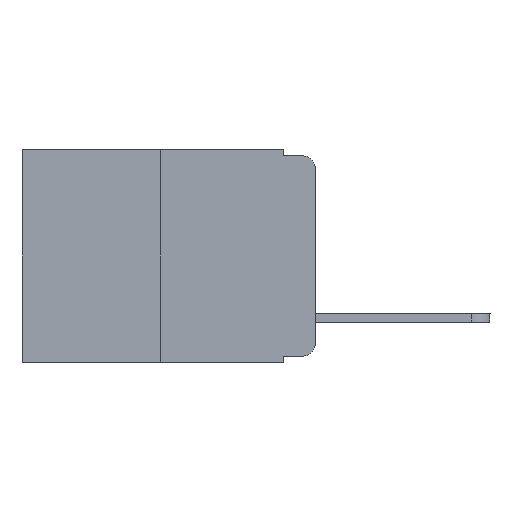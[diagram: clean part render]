
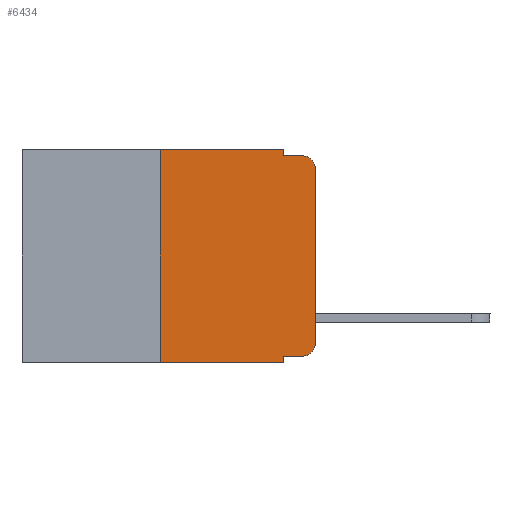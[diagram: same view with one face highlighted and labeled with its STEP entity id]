
A CAD part, left-side view. The second image highlights one B-rep face of the part: STEP entity #6434.
In plain terms, the highlighted planar face has unit normal (-1, 0, 0).
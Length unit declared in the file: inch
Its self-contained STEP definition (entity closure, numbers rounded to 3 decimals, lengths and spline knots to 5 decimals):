
#487 = DIRECTION ( 'NONE',  ( 0., -1., 0. ) ) ;
#492 = EDGE_CURVE ( 'NONE', #10321, #3591, #4329, .T. ) ;
#918 = VERTEX_POINT ( 'NONE', #18672 ) ;
#949 = EDGE_CURVE ( 'NONE', #10948, #1924, #9580, .T. ) ;
#983 = DIRECTION ( 'NONE',  ( 0., -1., 0. ) ) ;
#1165 = ORIENTED_EDGE ( 'NONE', *, *, #949, .T. ) ;
#1637 = CARTESIAN_POINT ( 'NONE',  ( 0., 0.473, -0.343 ) ) ;
#1924 = VERTEX_POINT ( 'NONE', #9732 ) ;
#2140 = AXIS2_PLACEMENT_3D ( 'NONE', #17310, #14210, #14512 ) ;
#2170 = DIRECTION ( 'NONE',  ( 0., -1., 0. ) ) ;
#2249 = DIRECTION ( 'NONE',  ( 1., 0., 0. ) ) ;
#2569 = LINE ( 'NONE', #8478, #4592 ) ;
#2744 = VECTOR ( 'NONE', #487, 39.37008 ) ;
#2855 = CARTESIAN_POINT ( 'NONE',  ( 0., 0.051, 0. ) ) ;
#3085 = ORIENTED_EDGE ( 'NONE', *, *, #8043, .F. ) ;
#3117 = ORIENTED_EDGE ( 'NONE', *, *, #14509, .F. ) ;
#3208 = LINE ( 'NONE', #7824, #2744 ) ;
#3591 = VERTEX_POINT ( 'NONE', #11490 ) ;
#3727 = LINE ( 'NONE', #6775, #8864 ) ;
#3771 = DIRECTION ( 'NONE',  ( 0., -1., 0. ) ) ;
#3957 = LINE ( 'NONE', #9946, #10611 ) ;
#4056 = EDGE_CURVE ( 'NONE', #10321, #16204, #3208, .T. ) ;
#4164 = ORIENTED_EDGE ( 'NONE', *, *, #4269, .T. ) ;
#4269 = EDGE_CURVE ( 'NONE', #16204, #10948, #13769, .T. ) ;
#4329 = LINE ( 'NONE', #2855, #8932 ) ;
#4592 = VECTOR ( 'NONE', #6805, 39.37008 ) ;
#4666 = CARTESIAN_POINT ( 'NONE',  ( 0., 0.02, -0.01 ) ) ;
#5198 = ORIENTED_EDGE ( 'NONE', *, *, #4056, .T. ) ;
#5773 = CARTESIAN_POINT ( 'NONE',  ( 0., 0.02, -0.03 ) ) ;
#6434 = ADVANCED_FACE ( 'NONE', ( #17172 ), #17071, .F. ) ;
#6484 = CARTESIAN_POINT ( 'NONE',  ( 0., 0., -0.313 ) ) ;
#6775 = CARTESIAN_POINT ( 'NONE',  ( 0., 0.25, 0. ) ) ;
#6805 = DIRECTION ( 'NONE',  ( 0., 0., -1. ) ) ;
#6868 = DIRECTION ( 'NONE',  ( 0., 0., -1. ) ) ;
#7388 = DIRECTION ( 'NONE',  ( 0., 0., -1. ) ) ;
#7522 = ORIENTED_EDGE ( 'NONE', *, *, #11802, .T. ) ;
#7824 = CARTESIAN_POINT ( 'NONE',  ( 0., 0.051, -0.333 ) ) ;
#8043 = EDGE_CURVE ( 'NONE', #10575, #12401, #3727, .T. ) ;
#8162 = CARTESIAN_POINT ( 'NONE',  ( 0., 0.473, 0. ) ) ;
#8204 = CARTESIAN_POINT ( 'NONE',  ( 0., 0., 0. ) ) ;
#8478 = CARTESIAN_POINT ( 'NONE',  ( 0., 0.051, 0. ) ) ;
#8864 = VECTOR ( 'NONE', #18920, 39.37008 ) ;
#8932 = VECTOR ( 'NONE', #7388, 39.37008 ) ;
#9501 = EDGE_CURVE ( 'NONE', #918, #12159, #2569, .T. ) ;
#9580 = LINE ( 'NONE', #8204, #13070 ) ;
#9732 = CARTESIAN_POINT ( 'NONE',  ( 0., 0., -0.03 ) ) ;
#9883 = CARTESIAN_POINT ( 'NONE',  ( 0., 0.051, -0.333 ) ) ;
#9946 = CARTESIAN_POINT ( 'NONE',  ( 0., 0.051, -0.01 ) ) ;
#10044 = LINE ( 'NONE', #16098, #13694 ) ;
#10305 = ORIENTED_EDGE ( 'NONE', *, *, #15652, .F. ) ;
#10321 = VERTEX_POINT ( 'NONE', #9883 ) ;
#10575 = VERTEX_POINT ( 'NONE', #16515 ) ;
#10611 = VECTOR ( 'NONE', #983, 39.37008 ) ;
#10948 = VERTEX_POINT ( 'NONE', #6484 ) ;
#11096 = ORIENTED_EDGE ( 'NONE', *, *, #9501, .F. ) ;
#11490 = CARTESIAN_POINT ( 'NONE',  ( 0., 0.051, -0.343 ) ) ;
#11598 = DIRECTION ( 'NONE',  ( -1., 0., 0. ) ) ;
#11802 = EDGE_CURVE ( 'NONE', #10575, #3591, #15707, .T. ) ;
#12159 = VERTEX_POINT ( 'NONE', #18313 ) ;
#12401 = VERTEX_POINT ( 'NONE', #14627 ) ;
#12628 = AXIS2_PLACEMENT_3D ( 'NONE', #8162, #2249, #15972 ) ;
#13070 = VECTOR ( 'NONE', #15519, 39.37008 ) ;
#13440 = AXIS2_PLACEMENT_3D ( 'NONE', #5773, #11598, #6868 ) ;
#13694 = VECTOR ( 'NONE', #2170, 39.37008 ) ;
#13769 = CIRCLE ( 'NONE', #2140, 0.02 ) ;
#14210 = DIRECTION ( 'NONE',  ( -1., 0., 0. ) ) ;
#14509 = EDGE_CURVE ( 'NONE', #12401, #918, #10044, .T. ) ;
#14512 = DIRECTION ( 'NONE',  ( 0., 0., -1. ) ) ;
#14543 = ORIENTED_EDGE ( 'NONE', *, *, #15995, .T. ) ;
#14627 = CARTESIAN_POINT ( 'NONE',  ( 0., 0.25, 0. ) ) ;
#14803 = CARTESIAN_POINT ( 'NONE',  ( 0., 0.02, -0.333 ) ) ;
#15064 = VERTEX_POINT ( 'NONE', #4666 ) ;
#15519 = DIRECTION ( 'NONE',  ( 0., 0., 1. ) ) ;
#15652 = EDGE_CURVE ( 'NONE', #12159, #15064, #3957, .T. ) ;
#15707 = LINE ( 'NONE', #1637, #18948 ) ;
#15752 = ORIENTED_EDGE ( 'NONE', *, *, #492, .F. ) ;
#15972 = DIRECTION ( 'NONE',  ( 0., 0., -1. ) ) ;
#15995 = EDGE_CURVE ( 'NONE', #1924, #15064, #16001, .T. ) ;
#16001 = CIRCLE ( 'NONE', #13440, 0.02 ) ;
#16098 = CARTESIAN_POINT ( 'NONE',  ( 0., 0.473, 0. ) ) ;
#16204 = VERTEX_POINT ( 'NONE', #14803 ) ;
#16515 = CARTESIAN_POINT ( 'NONE',  ( 0., 0.25, -0.343 ) ) ;
#17071 = PLANE ( 'NONE',  #12628 ) ;
#17172 = FACE_OUTER_BOUND ( 'NONE', #18337, .T. ) ;
#17310 = CARTESIAN_POINT ( 'NONE',  ( 0., 0.02, -0.313 ) ) ;
#18313 = CARTESIAN_POINT ( 'NONE',  ( 0., 0.051, -0.01 ) ) ;
#18337 = EDGE_LOOP ( 'NONE', ( #1165, #14543, #10305, #11096, #3117, #3085, #7522, #15752, #5198, #4164 ) ) ;
#18672 = CARTESIAN_POINT ( 'NONE',  ( 0., 0.051, 0. ) ) ;
#18920 = DIRECTION ( 'NONE',  ( 0., 0., 1. ) ) ;
#18948 = VECTOR ( 'NONE', #3771, 39.37008 ) ;
